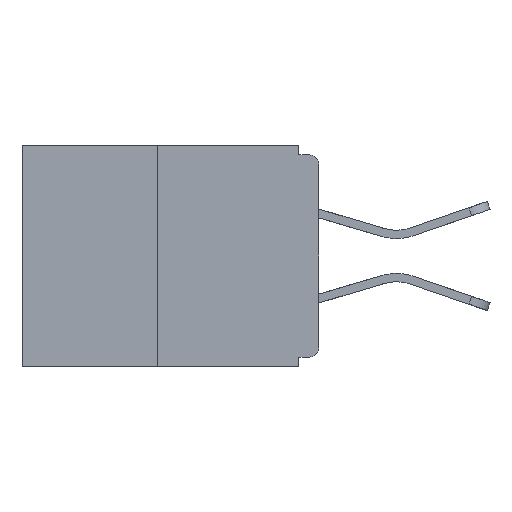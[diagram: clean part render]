
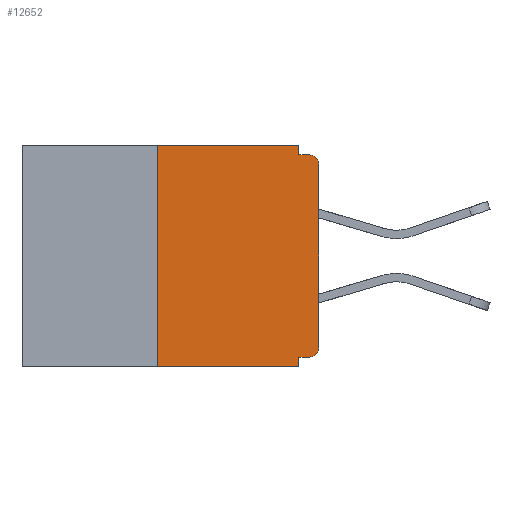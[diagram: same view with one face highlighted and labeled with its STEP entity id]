
A CAD part, left-side view. The second image highlights one B-rep face of the part: STEP entity #12652.
In plain terms, the highlighted planar face has unit normal (-1, 0, 0).
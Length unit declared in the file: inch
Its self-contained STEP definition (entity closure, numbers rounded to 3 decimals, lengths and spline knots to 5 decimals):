
#50 = ORIENTED_EDGE ( 'NONE', *, *, #13063, .F. ) ;
#77 = CARTESIAN_POINT ( 'NONE',  ( 0., 0.25, -0.343 ) ) ;
#222 = VECTOR ( 'NONE', #6106, 39.37008 ) ;
#310 = AXIS2_PLACEMENT_3D ( 'NONE', #9948, #3479, #12969 ) ;
#578 = EDGE_LOOP ( 'NONE', ( #10984, #6442, #2199, #50, #4130, #3657, #9939, #2228, #11992, #4923 ) ) ;
#631 = CARTESIAN_POINT ( 'NONE',  ( 0., 0.46, -0.343 ) ) ;
#752 = LINE ( 'NONE', #13184, #1582 ) ;
#1078 = VERTEX_POINT ( 'NONE', #7437 ) ;
#1134 = DIRECTION ( 'NONE',  ( 1., 0., 0. ) ) ;
#1230 = EDGE_CURVE ( 'NONE', #5459, #11526, #11310, .T. ) ;
#1582 = VECTOR ( 'NONE', #6941, 39.37008 ) ;
#2070 = PLANE ( 'NONE',  #3990 ) ;
#2109 = EDGE_CURVE ( 'NONE', #10852, #8323, #3004, .T. ) ;
#2199 = ORIENTED_EDGE ( 'NONE', *, *, #4886, .T. ) ;
#2228 = ORIENTED_EDGE ( 'NONE', *, *, #6745, .T. ) ;
#2417 = AXIS2_PLACEMENT_3D ( 'NONE', #6650, #7668, #4581 ) ;
#2882 = VERTEX_POINT ( 'NONE', #3465 ) ;
#3004 = LINE ( 'NONE', #4679, #222 ) ;
#3072 = LINE ( 'NONE', #631, #12849 ) ;
#3456 = CARTESIAN_POINT ( 'NONE',  ( 0., 0.25, 0. ) ) ;
#3465 = CARTESIAN_POINT ( 'NONE',  ( 0., 0.015, -0.328 ) ) ;
#3479 = DIRECTION ( 'NONE',  ( -1., 0., 0. ) ) ;
#3605 = CARTESIAN_POINT ( 'NONE',  ( 0., 0.031, 0. ) ) ;
#3657 = ORIENTED_EDGE ( 'NONE', *, *, #4056, .T. ) ;
#3990 = AXIS2_PLACEMENT_3D ( 'NONE', #7510, #1134, #9508 ) ;
#4056 = EDGE_CURVE ( 'NONE', #2882, #5459, #11237, .T. ) ;
#4130 = ORIENTED_EDGE ( 'NONE', *, *, #11400, .F. ) ;
#4236 = CARTESIAN_POINT ( 'NONE',  ( 0., 0.25, 0. ) ) ;
#4403 = DIRECTION ( 'NONE',  ( 0., -1., 0. ) ) ;
#4423 = CARTESIAN_POINT ( 'NONE',  ( 0., 0., -0.03 ) ) ;
#4424 = VERTEX_POINT ( 'NONE', #6532 ) ;
#4581 = DIRECTION ( 'NONE',  ( 0., 0., -1. ) ) ;
#4679 = CARTESIAN_POINT ( 'NONE',  ( 0., 0.031, 0. ) ) ;
#4798 = LINE ( 'NONE', #9134, #5125 ) ;
#4886 = EDGE_CURVE ( 'NONE', #9604, #1078, #3072, .T. ) ;
#4923 = ORIENTED_EDGE ( 'NONE', *, *, #2109, .F. ) ;
#4933 = CARTESIAN_POINT ( 'NONE',  ( 0., 0.031, -0.015 ) ) ;
#5125 = VECTOR ( 'NONE', #10215, 39.37008 ) ;
#5254 = VECTOR ( 'NONE', #9415, 39.37008 ) ;
#5459 = VERTEX_POINT ( 'NONE', #12379 ) ;
#5635 = EDGE_CURVE ( 'NONE', #9604, #12033, #12504, .T. ) ;
#6106 = DIRECTION ( 'NONE',  ( 0., 0., -1. ) ) ;
#6192 = EDGE_CURVE ( 'NONE', #12033, #10852, #12808, .T. ) ;
#6352 = CARTESIAN_POINT ( 'NONE',  ( 0., 0.015, -0.015 ) ) ;
#6442 = ORIENTED_EDGE ( 'NONE', *, *, #5635, .F. ) ;
#6532 = CARTESIAN_POINT ( 'NONE',  ( 0., 0.031, -0.328 ) ) ;
#6598 = DIRECTION ( 'NONE',  ( 0., 0., 1. ) ) ;
#6621 = VERTEX_POINT ( 'NONE', #6352 ) ;
#6650 = CARTESIAN_POINT ( 'NONE',  ( 0., 0.015, -0.03 ) ) ;
#6745 = EDGE_CURVE ( 'NONE', #11526, #6621, #6886, .T. ) ;
#6886 = CIRCLE ( 'NONE', #2417, 0.015 ) ;
#6941 = DIRECTION ( 'NONE',  ( 0., 0., -1. ) ) ;
#7437 = CARTESIAN_POINT ( 'NONE',  ( 0., 0.031, -0.343 ) ) ;
#7510 = CARTESIAN_POINT ( 'NONE',  ( 0., 0.46, 0. ) ) ;
#7668 = DIRECTION ( 'NONE',  ( -1., 0., 0. ) ) ;
#8065 = VECTOR ( 'NONE', #4403, 39.37008 ) ;
#8323 = VERTEX_POINT ( 'NONE', #4933 ) ;
#8680 = CARTESIAN_POINT ( 'NONE',  ( 0., 0., 0. ) ) ;
#9134 = CARTESIAN_POINT ( 'NONE',  ( 0., 0., -0.015 ) ) ;
#9415 = DIRECTION ( 'NONE',  ( 0., 1., 0. ) ) ;
#9508 = DIRECTION ( 'NONE',  ( 0., 0., -1. ) ) ;
#9604 = VERTEX_POINT ( 'NONE', #77 ) ;
#9737 = EDGE_CURVE ( 'NONE', #8323, #6621, #4798, .T. ) ;
#9852 = VECTOR ( 'NONE', #6598, 39.37008 ) ;
#9879 = VECTOR ( 'NONE', #11503, 39.37008 ) ;
#9939 = ORIENTED_EDGE ( 'NONE', *, *, #1230, .T. ) ;
#9948 = CARTESIAN_POINT ( 'NONE',  ( 0., 0.015, -0.313 ) ) ;
#10045 = DIRECTION ( 'NONE',  ( 0., -1., 0. ) ) ;
#10215 = DIRECTION ( 'NONE',  ( 0., -1., 0. ) ) ;
#10438 = CARTESIAN_POINT ( 'NONE',  ( 0., 0., -0.328 ) ) ;
#10561 = LINE ( 'NONE', #10438, #5254 ) ;
#10852 = VERTEX_POINT ( 'NONE', #3605 ) ;
#10857 = FACE_OUTER_BOUND ( 'NONE', #578, .T. ) ;
#10984 = ORIENTED_EDGE ( 'NONE', *, *, #6192, .F. ) ;
#11237 = CIRCLE ( 'NONE', #310, 0.015 ) ;
#11310 = LINE ( 'NONE', #8680, #9852 ) ;
#11400 = EDGE_CURVE ( 'NONE', #2882, #4424, #10561, .T. ) ;
#11503 = DIRECTION ( 'NONE',  ( 0., 0., 1. ) ) ;
#11526 = VERTEX_POINT ( 'NONE', #4423 ) ;
#11992 = ORIENTED_EDGE ( 'NONE', *, *, #9737, .F. ) ;
#12033 = VERTEX_POINT ( 'NONE', #3456 ) ;
#12379 = CARTESIAN_POINT ( 'NONE',  ( 0., 0., -0.313 ) ) ;
#12504 = LINE ( 'NONE', #4236, #9879 ) ;
#12652 = ADVANCED_FACE ( 'NONE', ( #10857 ), #2070, .F. ) ;
#12808 = LINE ( 'NONE', #12928, #8065 ) ;
#12849 = VECTOR ( 'NONE', #10045, 39.37008 ) ;
#12928 = CARTESIAN_POINT ( 'NONE',  ( 0., 0.46, 0. ) ) ;
#12969 = DIRECTION ( 'NONE',  ( 0., 0., -1. ) ) ;
#13063 = EDGE_CURVE ( 'NONE', #4424, #1078, #752, .T. ) ;
#13184 = CARTESIAN_POINT ( 'NONE',  ( 0., 0.031, -0.343 ) ) ;
